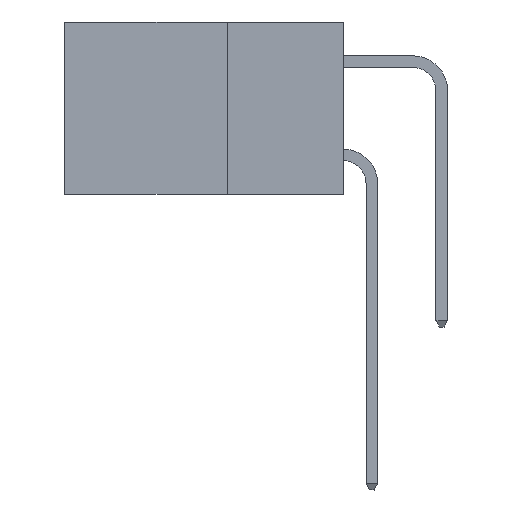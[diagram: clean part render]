
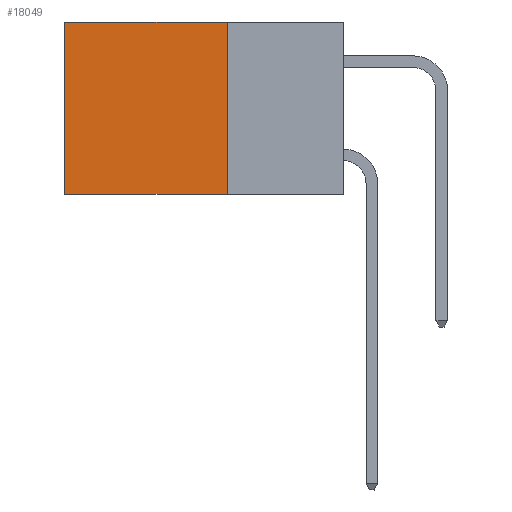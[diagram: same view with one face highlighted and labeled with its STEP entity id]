
A CAD part, left-side view. The second image highlights one B-rep face of the part: STEP entity #18049.
In plain terms, the highlighted planar face has unit normal (-1, 0, 0).
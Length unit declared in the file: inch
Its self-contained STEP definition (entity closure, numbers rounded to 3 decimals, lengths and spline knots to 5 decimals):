
#66 = VECTOR ( 'NONE', #8252, 39.37008 ) ;
#1109 = CARTESIAN_POINT ( 'NONE',  ( 0.2615, 0.6, -0.37 ) ) ;
#4346 = VECTOR ( 'NONE', #15993, 39.37008 ) ;
#5007 = EDGE_CURVE ( 'NONE', #18776, #23024, #22954, .T. ) ;
#5598 = CARTESIAN_POINT ( 'NONE',  ( 0.2615, 0.25, -0.37 ) ) ;
#6001 = DIRECTION ( 'NONE',  ( 1., 0., 0. ) ) ;
#6226 = ORIENTED_EDGE ( 'NONE', *, *, #13879, .T. ) ;
#6443 = CARTESIAN_POINT ( 'NONE',  ( 0.2615, 0.6, -0.37 ) ) ;
#6511 = CARTESIAN_POINT ( 'NONE',  ( 0.2615, 0.25, -0.37 ) ) ;
#6588 = CARTESIAN_POINT ( 'NONE',  ( 0.2615, 0.25, 0. ) ) ;
#7939 = PLANE ( 'NONE',  #17862 ) ;
#8250 = DIRECTION ( 'NONE',  ( 0., 0., -1. ) ) ;
#8252 = DIRECTION ( 'NONE',  ( 0., 0., -1. ) ) ;
#8997 = EDGE_CURVE ( 'NONE', #12621, #19603, #19423, .T. ) ;
#9038 = EDGE_LOOP ( 'NONE', ( #6226, #13911, #11066, #13344 ) ) ;
#9839 = DIRECTION ( 'NONE',  ( 0., 0., -1. ) ) ;
#9948 = FACE_OUTER_BOUND ( 'NONE', #9038, .T. ) ;
#10892 = VECTOR ( 'NONE', #8250, 39.37008 ) ;
#11066 = ORIENTED_EDGE ( 'NONE', *, *, #16881, .F. ) ;
#11781 = DIRECTION ( 'NONE',  ( 0., 1., 0. ) ) ;
#12621 = VERTEX_POINT ( 'NONE', #14575 ) ;
#13344 = ORIENTED_EDGE ( 'NONE', *, *, #8997, .T. ) ;
#13879 = EDGE_CURVE ( 'NONE', #19603, #23024, #17602, .T. ) ;
#13911 = ORIENTED_EDGE ( 'NONE', *, *, #5007, .F. ) ;
#14379 = VECTOR ( 'NONE', #11781, 39.37008 ) ;
#14575 = CARTESIAN_POINT ( 'NONE',  ( 0.2615, 0.25, 0. ) ) ;
#15585 = CARTESIAN_POINT ( 'NONE',  ( 0.2615, 0.25, -0.37 ) ) ;
#15923 = CARTESIAN_POINT ( 'NONE',  ( 0.2615, 0.25, -0.37 ) ) ;
#15993 = DIRECTION ( 'NONE',  ( 0., 1., 0. ) ) ;
#16881 = EDGE_CURVE ( 'NONE', #12621, #18776, #21192, .T. ) ;
#17602 = LINE ( 'NONE', #6443, #66 ) ;
#17862 = AXIS2_PLACEMENT_3D ( 'NONE', #15585, #6001, #9839 ) ;
#18049 = ADVANCED_FACE ( 'NONE', ( #9948 ), #7939, .F. ) ;
#18776 = VERTEX_POINT ( 'NONE', #5598 ) ;
#19333 = CARTESIAN_POINT ( 'NONE',  ( 0.2615, 0.6, 0. ) ) ;
#19423 = LINE ( 'NONE', #6588, #14379 ) ;
#19603 = VERTEX_POINT ( 'NONE', #19333 ) ;
#21192 = LINE ( 'NONE', #15923, #10892 ) ;
#22954 = LINE ( 'NONE', #6511, #4346 ) ;
#23024 = VERTEX_POINT ( 'NONE', #1109 ) ;
